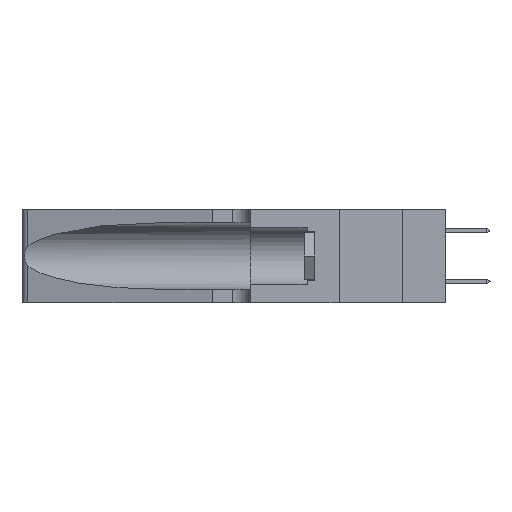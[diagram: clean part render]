
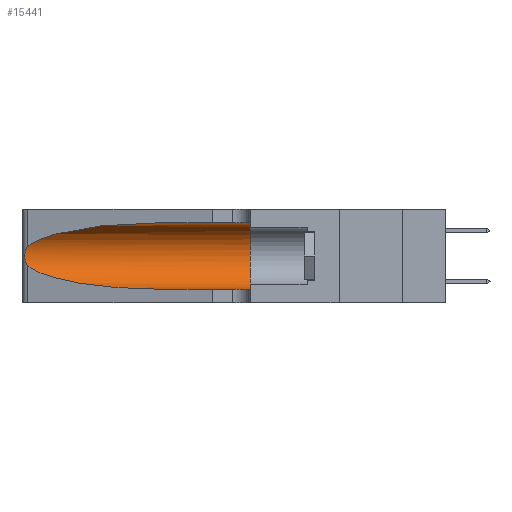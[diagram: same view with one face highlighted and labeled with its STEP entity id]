
A CAD part, left-side view. The second image highlights one B-rep face of the part: STEP entity #15441.
In plain terms, the highlighted cylindrical face has radius 3.308 mm (diameter 6.617 mm), a partial arc.
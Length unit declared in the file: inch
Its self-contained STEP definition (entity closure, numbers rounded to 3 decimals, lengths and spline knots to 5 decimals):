
#521 = CARTESIAN_POINT ( 'NONE',  ( 0.1305, 0.35, 0.05475 ) ) ;
#712 = CARTESIAN_POINT ( 'NONE',  ( 0.25856, 1.23593, 0.16098 ) ) ;
#1242 = ORIENTED_EDGE ( 'NONE', *, *, #10088, .F. ) ;
#1291 = EDGE_CURVE ( 'NONE', #13187, #12142, #13384, .T. ) ;
#1403 = DIRECTION ( 'NONE',  ( 0., 0., -1. ) ) ;
#1798 = FACE_OUTER_BOUND ( 'NONE', #5883, .T. ) ;
#2343 = LINE ( 'NONE', #23377, #18757 ) ;
#2824 = CARTESIAN_POINT ( 'NONE',  ( 0.25639, 1.23186, 0.15144 ) ) ;
#2969 = CARTESIAN_POINT ( 'NONE',  ( 0.1305, 0.72297, 0.31525 ) ) ;
#3365 = EDGE_CURVE ( 'NONE', #24090, #9609, #8388, .T. ) ;
#4995 = CARTESIAN_POINT ( 'NONE',  ( 0.25487, 1.22718, 0.14631 ) ) ;
#5147 = CARTESIAN_POINT ( 'NONE',  ( 0.25487, 1.22718, 0.22369 ) ) ;
#5268 = EDGE_CURVE ( 'NONE', #24090, #8759, #16123, .T. ) ;
#5604 = EDGE_CURVE ( 'NONE', #12142, #10852, #2343, .T. ) ;
#5838 = CIRCLE ( 'NONE', #20073, 0.13025 ) ;
#5883 = EDGE_LOOP ( 'NONE', ( #22217, #11810, #16905, #18070, #1242, #14656 ) ) ;
#5897 = CARTESIAN_POINT ( 'NONE',  ( 0.25639, 1.23184, 0.21858 ) ) ;
#6816 = CARTESIAN_POINT ( 'NONE',  ( 0.25487, 1.22718, 0.22369 ) ) ;
#6910 = CARTESIAN_POINT ( 'NONE',  ( 0.25854, 1.2359, 0.20912 ) ) ;
#8377 = DIRECTION ( 'NONE',  ( 0., 1., 0. ) ) ;
#8388 =( BOUNDED_CURVE ( )  B_SPLINE_CURVE ( 3, ( #2969, #15823, #17972, #5147 ),
 .UNSPECIFIED., .F., .T. ) 
 B_SPLINE_CURVE_WITH_KNOTS ( ( 4, 4 ),
 ( 1.5708, 2.84003 ),
 .UNSPECIFIED. ) 
 CURVE ( )  GEOMETRIC_REPRESENTATION_ITEM ( )  RATIONAL_B_SPLINE_CURVE ( ( 1., 0.87, 0.87, 1. ) ) 
 REPRESENTATION_ITEM ( '' )  );
#8759 = VERTEX_POINT ( 'NONE', #16710 ) ;
#9609 = VERTEX_POINT ( 'NONE', #6816 ) ;
#10082 = CARTESIAN_POINT ( 'NONE',  ( 0.25487, 1.22718, 0.14631 ) ) ;
#10088 = EDGE_CURVE ( 'NONE', #8759, #10852, #5838, .T. ) ;
#10408 = VECTOR ( 'NONE', #22137, 39.37008 ) ;
#10852 = VERTEX_POINT ( 'NONE', #521 ) ;
#11347 = CARTESIAN_POINT ( 'NONE',  ( 0.26075, 1.23896, 0.19203 ) ) ;
#11410 = CARTESIAN_POINT ( 'NONE',  ( 0.1305, 1.61858, 0.31525 ) ) ;
#11810 = ORIENTED_EDGE ( 'NONE', *, *, #14551, .T. ) ;
#12142 = VERTEX_POINT ( 'NONE', #25963 ) ;
#13187 = VERTEX_POINT ( 'NONE', #10082 ) ;
#13384 =( BOUNDED_CURVE ( )  B_SPLINE_CURVE ( 3, ( #21569, #21658, #26664, #21345 ),
 .UNSPECIFIED., .F., .F. ) 
 B_SPLINE_CURVE_WITH_KNOTS ( ( 4, 4 ),
 ( 3.44316, 4.71239 ),
 .UNSPECIFIED. ) 
 CURVE ( )  GEOMETRIC_REPRESENTATION_ITEM ( )  RATIONAL_B_SPLINE_CURVE ( ( 1., 0.87, 0.87, 1. ) ) 
 REPRESENTATION_ITEM ( '' )  );
#13526 = CARTESIAN_POINT ( 'NONE',  ( 0.26017, 1.23833, 0.17102 ) ) ;
#14238 = DIRECTION ( 'NONE',  ( 0., -1., 0. ) ) ;
#14551 = EDGE_CURVE ( 'NONE', #9609, #13187, #16315, .T. ) ;
#14656 = ORIENTED_EDGE ( 'NONE', *, *, #5268, .F. ) ;
#15441 = ADVANCED_FACE ( 'NONE', ( #1798 ), #17543, .F. ) ;
#15673 = CARTESIAN_POINT ( 'NONE',  ( 0.25789, 1.23486, 0.15765 ) ) ;
#15823 = CARTESIAN_POINT ( 'NONE',  ( 0.18966, 0.96281, 0.31525 ) ) ;
#16123 = LINE ( 'NONE', #11410, #10408 ) ;
#16315 = B_SPLINE_CURVE_WITH_KNOTS ( 'NONE', 3,
 ( #16593, #18716, #5897, #20841, #6910, #24112, #11347, #26236, #13526, #712, #15673, #2824, #17820, #4995 ),
 .UNSPECIFIED., .F., .F.,
 ( 4, 2, 2, 2, 2, 2, 4 ),
 ( 0., 0.00027, 0.00053, 0.00107, 0.0016, 0.00187, 0.00214 ),
 .UNSPECIFIED. ) ;
#16593 = CARTESIAN_POINT ( 'NONE',  ( 0.25487, 1.22718, 0.22369 ) ) ;
#16710 = CARTESIAN_POINT ( 'NONE',  ( 0.1305, 0.35, 0.31525 ) ) ;
#16905 = ORIENTED_EDGE ( 'NONE', *, *, #1291, .T. ) ;
#17543 = CYLINDRICAL_SURFACE ( 'NONE', #22997, 0.13025 ) ;
#17820 = CARTESIAN_POINT ( 'NONE',  ( 0.25555, 1.22993, 0.14849 ) ) ;
#17972 = CARTESIAN_POINT ( 'NONE',  ( 0.2373, 1.15595, 0.28018 ) ) ;
#18070 = ORIENTED_EDGE ( 'NONE', *, *, #5604, .T. ) ;
#18716 = CARTESIAN_POINT ( 'NONE',  ( 0.25555, 1.22994, 0.2215 ) ) ;
#18757 = VECTOR ( 'NONE', #25518, 39.37008 ) ;
#20073 = AXIS2_PLACEMENT_3D ( 'NONE', #21178, #8377, #23310 ) ;
#20841 = CARTESIAN_POINT ( 'NONE',  ( 0.25787, 1.23484, 0.2124 ) ) ;
#21178 = CARTESIAN_POINT ( 'NONE',  ( 0.1305, 0.35, 0.185 ) ) ;
#21345 = CARTESIAN_POINT ( 'NONE',  ( 0.1305, 0.72297, 0.05475 ) ) ;
#21569 = CARTESIAN_POINT ( 'NONE',  ( 0.25487, 1.22718, 0.14631 ) ) ;
#21658 = CARTESIAN_POINT ( 'NONE',  ( 0.2373, 1.15595, 0.08982 ) ) ;
#22137 = DIRECTION ( 'NONE',  ( 0., -1., 0. ) ) ;
#22217 = ORIENTED_EDGE ( 'NONE', *, *, #3365, .T. ) ;
#22997 = AXIS2_PLACEMENT_3D ( 'NONE', #26942, #14238, #1403 ) ;
#23310 = DIRECTION ( 'NONE',  ( 0., 0., 1. ) ) ;
#23377 = CARTESIAN_POINT ( 'NONE',  ( 0.1305, 1.61858, 0.05475 ) ) ;
#24090 = VERTEX_POINT ( 'NONE', #24793 ) ;
#24112 = CARTESIAN_POINT ( 'NONE',  ( 0.26018, 1.23835, 0.19895 ) ) ;
#24793 = CARTESIAN_POINT ( 'NONE',  ( 0.1305, 0.72297, 0.31525 ) ) ;
#25518 = DIRECTION ( 'NONE',  ( 0., -1., 0. ) ) ;
#25963 = CARTESIAN_POINT ( 'NONE',  ( 0.1305, 0.72297, 0.05475 ) ) ;
#26236 = CARTESIAN_POINT ( 'NONE',  ( 0.26075, 1.23896, 0.178 ) ) ;
#26664 = CARTESIAN_POINT ( 'NONE',  ( 0.18966, 0.96281, 0.05475 ) ) ;
#26942 = CARTESIAN_POINT ( 'NONE',  ( 0.1305, 1.61858, 0.185 ) ) ;
